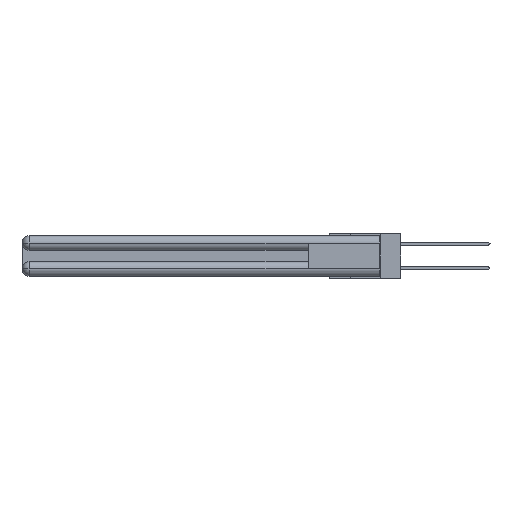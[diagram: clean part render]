
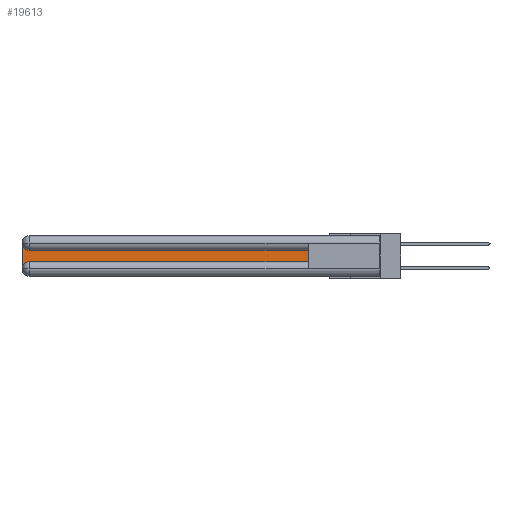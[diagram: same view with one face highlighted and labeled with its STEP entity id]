
A CAD part, left-side view. The second image highlights one B-rep face of the part: STEP entity #19613.
In plain terms, the highlighted planar face has unit normal (-1, 0, 0).
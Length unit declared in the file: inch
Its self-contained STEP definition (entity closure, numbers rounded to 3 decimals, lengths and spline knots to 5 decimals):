
#89 = LINE ( 'NONE', #5351, #27756 ) ;
#1790 = CARTESIAN_POINT ( 'NONE',  ( 0.075, 2.94, -0.2175 ) ) ;
#1886 = VECTOR ( 'NONE', #6000, 39.37008 ) ;
#2442 = CARTESIAN_POINT ( 'NONE',  ( 0.075, 0.6, -0.2175 ) ) ;
#2616 = VERTEX_POINT ( 'NONE', #12772 ) ;
#3408 = ORIENTED_EDGE ( 'NONE', *, *, #14072, .T. ) ;
#3807 = LINE ( 'NONE', #25519, #10906 ) ;
#3991 = DIRECTION ( 'NONE',  ( 1., 0., 0. ) ) ;
#5351 = CARTESIAN_POINT ( 'NONE',  ( 0.075, 0.6, -0.2175 ) ) ;
#5556 = DIRECTION ( 'NONE',  ( 0., 0., -1. ) ) ;
#5792 = AXIS2_PLACEMENT_3D ( 'NONE', #29108, #13119, #5556 ) ;
#6000 = DIRECTION ( 'NONE',  ( 0., 0., 1. ) ) ;
#6371 = ORIENTED_EDGE ( 'NONE', *, *, #17792, .T. ) ;
#7345 = FACE_OUTER_BOUND ( 'NONE', #8263, .T. ) ;
#7636 = CARTESIAN_POINT ( 'NONE',  ( 0.075, 2.94, -0.2775 ) ) ;
#8125 = PLANE ( 'NONE',  #5792 ) ;
#8263 = EDGE_LOOP ( 'NONE', ( #6371, #16491, #32267, #17105, #3408, #23045 ) ) ;
#9122 = LINE ( 'NONE', #11128, #33879 ) ;
#10298 = DIRECTION ( 'NONE',  ( 1., 0., 0. ) ) ;
#10621 = CARTESIAN_POINT ( 'NONE',  ( 0.075, 3., -0.2775 ) ) ;
#10883 = EDGE_CURVE ( 'NONE', #29955, #14406, #32150, .T. ) ;
#10906 = VECTOR ( 'NONE', #20195, 39.37008 ) ;
#11128 = CARTESIAN_POINT ( 'NONE',  ( 0.075, 0.6, -0.1225 ) ) ;
#12772 = CARTESIAN_POINT ( 'NONE',  ( 0.075, 0.6, -0.1225 ) ) ;
#13119 = DIRECTION ( 'NONE',  ( 1., 0., 0. ) ) ;
#14072 = EDGE_CURVE ( 'NONE', #32368, #29637, #89, .T. ) ;
#14406 = VERTEX_POINT ( 'NONE', #28316 ) ;
#16491 = ORIENTED_EDGE ( 'NONE', *, *, #10883, .T. ) ;
#16908 = LINE ( 'NONE', #21989, #1886 ) ;
#17105 = ORIENTED_EDGE ( 'NONE', *, *, #17297, .T. ) ;
#17297 = EDGE_CURVE ( 'NONE', #32790, #32368, #21295, .T. ) ;
#17792 = EDGE_CURVE ( 'NONE', #2616, #29955, #9122, .T. ) ;
#18533 = DIRECTION ( 'NONE',  ( 0., -1., 0. ) ) ;
#18933 = AXIS2_PLACEMENT_3D ( 'NONE', #7636, #10298, #29072 ) ;
#19613 = ADVANCED_FACE ( 'NONE', ( #7345 ), #8125, .F. ) ;
#20195 = DIRECTION ( 'NONE',  ( 0., 0., -1. ) ) ;
#21295 = CIRCLE ( 'NONE', #18933, 0.06 ) ;
#21536 = DIRECTION ( 'NONE',  ( 0., 1., 0. ) ) ;
#21989 = CARTESIAN_POINT ( 'NONE',  ( 0.075, 0.6, -0.2175 ) ) ;
#23045 = ORIENTED_EDGE ( 'NONE', *, *, #24546, .T. ) ;
#24546 = EDGE_CURVE ( 'NONE', #29637, #2616, #16908, .T. ) ;
#24928 = CARTESIAN_POINT ( 'NONE',  ( 0.075, 2.94, -0.1225 ) ) ;
#25519 = CARTESIAN_POINT ( 'NONE',  ( 0.075, 3., -0.2175 ) ) ;
#26779 = EDGE_CURVE ( 'NONE', #14406, #32790, #3807, .T. ) ;
#27756 = VECTOR ( 'NONE', #18533, 39.37008 ) ;
#28312 = AXIS2_PLACEMENT_3D ( 'NONE', #30722, #3991, #33165 ) ;
#28316 = CARTESIAN_POINT ( 'NONE',  ( 0.075, 3., -0.0625 ) ) ;
#29072 = DIRECTION ( 'NONE',  ( 0., 0., -1. ) ) ;
#29108 = CARTESIAN_POINT ( 'NONE',  ( 0.075, 3., -0.1225 ) ) ;
#29637 = VERTEX_POINT ( 'NONE', #2442 ) ;
#29955 = VERTEX_POINT ( 'NONE', #24928 ) ;
#30722 = CARTESIAN_POINT ( 'NONE',  ( 0.075, 2.94, -0.0625 ) ) ;
#32150 = CIRCLE ( 'NONE', #28312, 0.06 ) ;
#32267 = ORIENTED_EDGE ( 'NONE', *, *, #26779, .T. ) ;
#32368 = VERTEX_POINT ( 'NONE', #1790 ) ;
#32790 = VERTEX_POINT ( 'NONE', #10621 ) ;
#33165 = DIRECTION ( 'NONE',  ( 0., 0., -1. ) ) ;
#33879 = VECTOR ( 'NONE', #21536, 39.37008 ) ;
